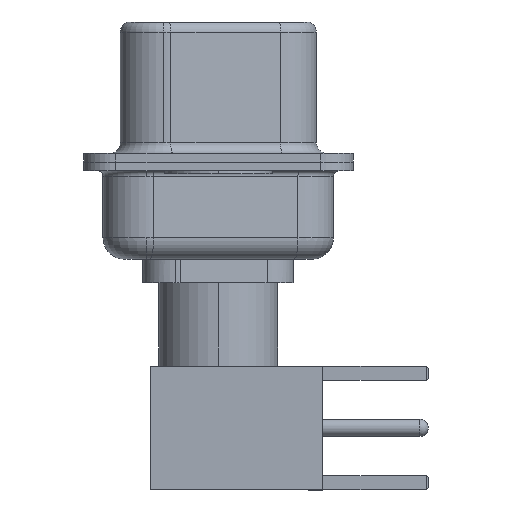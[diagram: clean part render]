
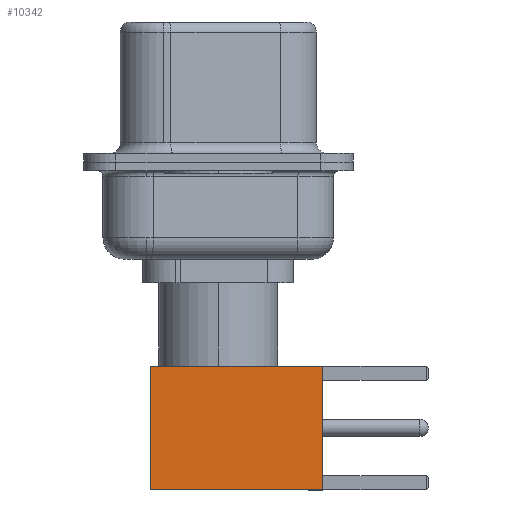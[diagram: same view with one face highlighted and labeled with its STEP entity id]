
A CAD part, left-side view. The second image highlights one B-rep face of the part: STEP entity #10342.
In plain terms, the highlighted face is planar.
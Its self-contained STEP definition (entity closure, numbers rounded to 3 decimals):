
#6 = VERTEX_POINT ( 'NONE', #10920 ) ;
#173 = EDGE_CURVE ( 'NONE', #6, #6126, #8875, .T. ) ;
#865 = FACE_OUTER_BOUND ( 'NONE', #9652, .T. ) ;
#1840 = DIRECTION ( 'NONE',  ( 0., 1., 0. ) ) ;
#1858 = CARTESIAN_POINT ( 'NONE',  ( 0., 2.875, 8. ) ) ;
#2210 = AXIS2_PLACEMENT_3D ( 'NONE', #15462, #1840, #10497 ) ;
#2345 = CARTESIAN_POINT ( 'NONE',  ( -2.875, 2.875, 0. ) ) ;
#3655 = EDGE_CURVE ( 'NONE', #6126, #12227, #12504, .T. ) ;
#4170 = ORIENTED_EDGE ( 'NONE', *, *, #173, .T. ) ;
#5426 = CARTESIAN_POINT ( 'NONE',  ( 0., 2.875, 0. ) ) ;
#5478 = VECTOR ( 'NONE', #10362, 1000. ) ;
#5510 = ORIENTED_EDGE ( 'NONE', *, *, #8592, .F. ) ;
#5639 = CARTESIAN_POINT ( 'NONE',  ( -2.875, 2.875, 8. ) ) ;
#6126 = VERTEX_POINT ( 'NONE', #14192 ) ;
#7674 = DIRECTION ( 'NONE',  ( 0., 0., -1. ) ) ;
#8592 = EDGE_CURVE ( 'NONE', #6, #13466, #10512, .T. ) ;
#8875 = LINE ( 'NONE', #13697, #10849 ) ;
#8990 = EDGE_CURVE ( 'NONE', #13466, #12227, #9441, .T. ) ;
#9441 = LINE ( 'NONE', #14264, #12836 ) ;
#9652 = EDGE_LOOP ( 'NONE', ( #4170, #10688, #12106, #5510 ) ) ;
#10342 = ADVANCED_FACE ( 'NONE', ( #865 ), #10348, .T. ) ;
#10348 = PLANE ( 'NONE',  #2210 ) ;
#10362 = DIRECTION ( 'NONE',  ( -1., 0., 0. ) ) ;
#10497 = DIRECTION ( 'NONE',  ( 0., 0., 1. ) ) ;
#10512 = LINE ( 'NONE', #1858, #5478 ) ;
#10688 = ORIENTED_EDGE ( 'NONE', *, *, #3655, .T. ) ;
#10849 = VECTOR ( 'NONE', #7674, 1000. ) ;
#10920 = CARTESIAN_POINT ( 'NONE',  ( 2.875, 2.875, 8. ) ) ;
#12106 = ORIENTED_EDGE ( 'NONE', *, *, #8990, .F. ) ;
#12227 = VERTEX_POINT ( 'NONE', #2345 ) ;
#12340 = DIRECTION ( 'NONE',  ( -1., 0., 0. ) ) ;
#12504 = LINE ( 'NONE', #5426, #15115 ) ;
#12836 = VECTOR ( 'NONE', #13060, 1000. ) ;
#13060 = DIRECTION ( 'NONE',  ( 0., 0., -1. ) ) ;
#13466 = VERTEX_POINT ( 'NONE', #5639 ) ;
#13697 = CARTESIAN_POINT ( 'NONE',  ( 2.875, 2.875, 0. ) ) ;
#14192 = CARTESIAN_POINT ( 'NONE',  ( 2.875, 2.875, 0. ) ) ;
#14264 = CARTESIAN_POINT ( 'NONE',  ( -2.875, 2.875, 0. ) ) ;
#15115 = VECTOR ( 'NONE', #12340, 1000. ) ;
#15462 = CARTESIAN_POINT ( 'NONE',  ( 2.875, 2.875, 0. ) ) ;
